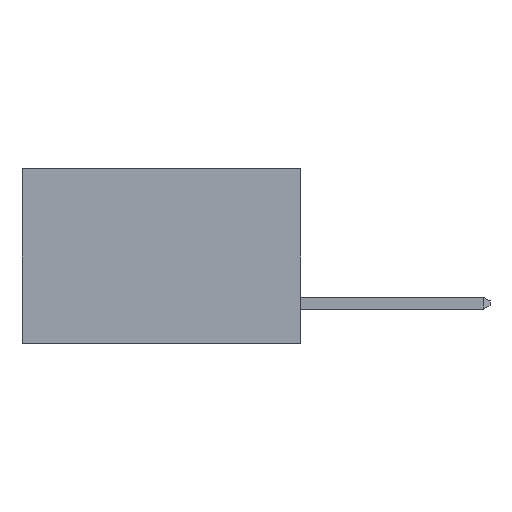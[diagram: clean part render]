
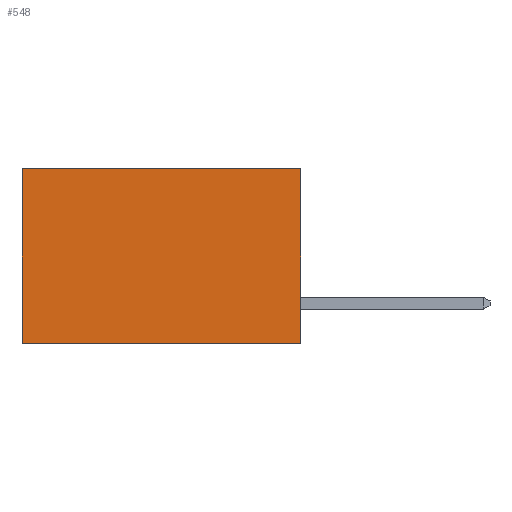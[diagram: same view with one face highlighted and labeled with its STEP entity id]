
A CAD part, left-side view. The second image highlights one B-rep face of the part: STEP entity #548.
In plain terms, the highlighted planar face has unit normal (-1, 0, 0).
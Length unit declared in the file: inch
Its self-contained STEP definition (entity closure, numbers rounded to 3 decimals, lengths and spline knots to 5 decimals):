
#205 = CARTESIAN_POINT ( 'NONE',  ( 0.277, 0.59, -0.37 ) ) ;
#394 = ORIENTED_EDGE ( 'NONE', *, *, #5155, .F. ) ;
#547 = VERTEX_POINT ( 'NONE', #2222 ) ;
#548 = ADVANCED_FACE ( 'NONE', ( #6519 ), #5724, .F. ) ;
#1324 = LINE ( 'NONE', #7540, #7505 ) ;
#1697 = VECTOR ( 'NONE', #2794, 39.37008 ) ;
#1906 = LINE ( 'NONE', #3512, #6552 ) ;
#2042 = CARTESIAN_POINT ( 'NONE',  ( 0.277, 0.59, 0. ) ) ;
#2222 = CARTESIAN_POINT ( 'NONE',  ( 0.277, 0., -0.37 ) ) ;
#2374 = EDGE_CURVE ( 'NONE', #6767, #547, #7354, .T. ) ;
#2794 = DIRECTION ( 'NONE',  ( 0., 1., 0. ) ) ;
#3295 = CARTESIAN_POINT ( 'NONE',  ( 0.277, 0., 0. ) ) ;
#3416 = LINE ( 'NONE', #3295, #1697 ) ;
#3512 = CARTESIAN_POINT ( 'NONE',  ( 0.277, 0., -0.37 ) ) ;
#3656 = EDGE_CURVE ( 'NONE', #5763, #4276, #1324, .T. ) ;
#3659 = DIRECTION ( 'NONE',  ( 0., 0., -1. ) ) ;
#3956 = DIRECTION ( 'NONE',  ( 1., 0., 0. ) ) ;
#4276 = VERTEX_POINT ( 'NONE', #205 ) ;
#4544 = DIRECTION ( 'NONE',  ( 0., 0., -1. ) ) ;
#4553 = CARTESIAN_POINT ( 'NONE',  ( 0.277, 0., 0. ) ) ;
#5054 = DIRECTION ( 'NONE',  ( 0., 1., 0. ) ) ;
#5155 = EDGE_CURVE ( 'NONE', #547, #4276, #1906, .T. ) ;
#5167 = EDGE_CURVE ( 'NONE', #6767, #5763, #3416, .T. ) ;
#5432 = ORIENTED_EDGE ( 'NONE', *, *, #2374, .F. ) ;
#5604 = EDGE_LOOP ( 'NONE', ( #6759, #394, #5432, #6927 ) ) ;
#5724 = PLANE ( 'NONE',  #6717 ) ;
#5763 = VERTEX_POINT ( 'NONE', #2042 ) ;
#5882 = VECTOR ( 'NONE', #3659, 39.37008 ) ;
#6519 = FACE_OUTER_BOUND ( 'NONE', #5604, .T. ) ;
#6552 = VECTOR ( 'NONE', #5054, 39.37008 ) ;
#6717 = AXIS2_PLACEMENT_3D ( 'NONE', #7370, #3956, #4544 ) ;
#6759 = ORIENTED_EDGE ( 'NONE', *, *, #3656, .T. ) ;
#6767 = VERTEX_POINT ( 'NONE', #4553 ) ;
#6927 = ORIENTED_EDGE ( 'NONE', *, *, #5167, .T. ) ;
#7354 = LINE ( 'NONE', #7695, #5882 ) ;
#7370 = CARTESIAN_POINT ( 'NONE',  ( 0.277, 0., -0.37 ) ) ;
#7505 = VECTOR ( 'NONE', #7601, 39.37008 ) ;
#7540 = CARTESIAN_POINT ( 'NONE',  ( 0.277, 0.59, -0.37 ) ) ;
#7601 = DIRECTION ( 'NONE',  ( 0., 0., -1. ) ) ;
#7695 = CARTESIAN_POINT ( 'NONE',  ( 0.277, 0., -0.37 ) ) ;
